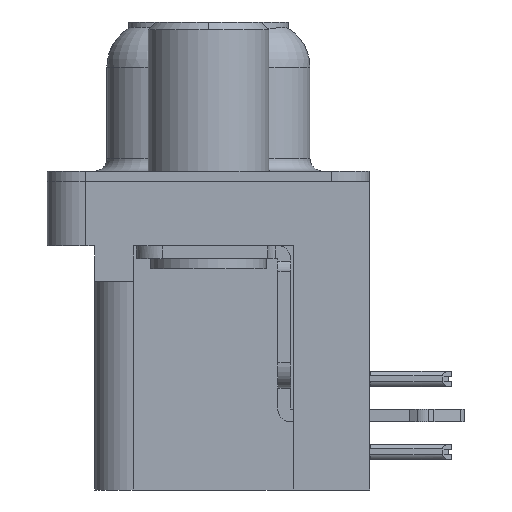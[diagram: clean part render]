
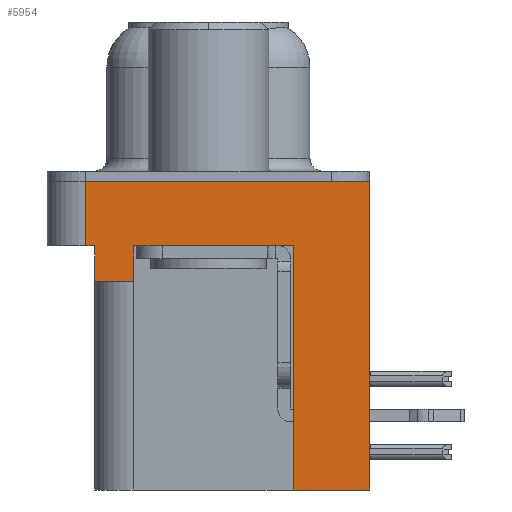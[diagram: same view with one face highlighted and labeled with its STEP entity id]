
A CAD part, left-side view. The second image highlights one B-rep face of the part: STEP entity #5954.
In plain terms, the highlighted planar face has unit normal (-1, 0, 0).
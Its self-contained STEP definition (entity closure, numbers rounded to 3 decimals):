
#320 = VECTOR ( 'NONE', #23377, 1000. ) ;
#1437 = VECTOR ( 'NONE', #6944, 1000. ) ;
#1944 = VECTOR ( 'NONE', #24552, 1000. ) ;
#2873 = AXIS2_PLACEMENT_3D ( 'NONE', #18936, #24991, #16897 ) ;
#3666 = VECTOR ( 'NONE', #25841, 1000. ) ;
#4092 = CARTESIAN_POINT ( 'NONE',  ( -2.935, -3.295, -12. ) ) ;
#4258 = VECTOR ( 'NONE', #9089, 1000. ) ;
#4611 = VECTOR ( 'NONE', #23401, 1000. ) ;
#4792 = EDGE_CURVE ( 'NONE', #22849, #14926, #17560, .T. ) ;
#5066 = VECTOR ( 'NONE', #19880, 1000. ) ;
#5247 = ORIENTED_EDGE ( 'NONE', *, *, #17541, .F. ) ;
#5258 = CARTESIAN_POINT ( 'NONE',  ( -2.935, 4.775, 0. ) ) ;
#5954 = ADVANCED_FACE ( 'NONE', ( #20139 ), #21109, .T. ) ;
#6425 = ORIENTED_EDGE ( 'NONE', *, *, #15629, .F. ) ;
#6846 = VERTEX_POINT ( 'NONE', #7409 ) ;
#6944 = DIRECTION ( 'NONE',  ( 0., 0., 1. ) ) ;
#7409 = CARTESIAN_POINT ( 'NONE',  ( -2.935, 4.425, -2.5 ) ) ;
#8389 = DIRECTION ( 'NONE',  ( 0., -1., 0. ) ) ;
#8557 = CARTESIAN_POINT ( 'NONE',  ( -2.935, -6.275, -12. ) ) ;
#9089 = DIRECTION ( 'NONE',  ( 0., 0., 1. ) ) ;
#9240 = ORIENTED_EDGE ( 'NONE', *, *, #19160, .T. ) ;
#9241 = CARTESIAN_POINT ( 'NONE',  ( -2.935, 4.425, -3.9 ) ) ;
#9741 = CARTESIAN_POINT ( 'NONE',  ( -2.935, -6.275, -2.5 ) ) ;
#9823 = DIRECTION ( 'NONE',  ( 0., 0., 1. ) ) ;
#10396 = ORIENTED_EDGE ( 'NONE', *, *, #18893, .T. ) ;
#10467 = CARTESIAN_POINT ( 'NONE',  ( -2.935, -6.275, 0. ) ) ;
#10673 = LINE ( 'NONE', #23793, #5066 ) ;
#10853 = CARTESIAN_POINT ( 'NONE',  ( -2.935, 2.895, -3.9 ) ) ;
#10885 = LINE ( 'NONE', #19027, #4611 ) ;
#11227 = ORIENTED_EDGE ( 'NONE', *, *, #20827, .F. ) ;
#11472 = LINE ( 'NONE', #19969, #1944 ) ;
#12484 = LINE ( 'NONE', #4092, #21060 ) ;
#12675 = CARTESIAN_POINT ( 'NONE',  ( -2.935, -6.275, 0. ) ) ;
#12857 = LINE ( 'NONE', #15121, #320 ) ;
#13091 = ORIENTED_EDGE ( 'NONE', *, *, #19710, .F. ) ;
#13749 = VECTOR ( 'NONE', #8389, 1000. ) ;
#14563 = DIRECTION ( 'NONE',  ( 0., 1., 0. ) ) ;
#14926 = VERTEX_POINT ( 'NONE', #24550 ) ;
#15121 = CARTESIAN_POINT ( 'NONE',  ( -2.935, -3.295, -12. ) ) ;
#15629 = EDGE_CURVE ( 'NONE', #22641, #6846, #24526, .T. ) ;
#16434 = LINE ( 'NONE', #12675, #13749 ) ;
#16897 = DIRECTION ( 'NONE',  ( 0., 0., 1. ) ) ;
#16963 = ORIENTED_EDGE ( 'NONE', *, *, #4792, .T. ) ;
#17541 = EDGE_CURVE ( 'NONE', #22849, #22641, #10885, .T. ) ;
#17560 = LINE ( 'NONE', #10853, #3666 ) ;
#17630 = VERTEX_POINT ( 'NONE', #10467 ) ;
#17770 = ORIENTED_EDGE ( 'NONE', *, *, #19288, .T. ) ;
#18009 = LINE ( 'NONE', #9741, #19653 ) ;
#18197 = EDGE_CURVE ( 'NONE', #25537, #19764, #12857, .T. ) ;
#18319 = VERTEX_POINT ( 'NONE', #5258 ) ;
#18652 = EDGE_CURVE ( 'NONE', #26982, #18319, #25738, .T. ) ;
#18893 = EDGE_CURVE ( 'NONE', #21520, #17630, #18009, .T. ) ;
#18936 = CARTESIAN_POINT ( 'NONE',  ( -2.935, -6.275, -2.5 ) ) ;
#19027 = CARTESIAN_POINT ( 'NONE',  ( -2.935, 4.425, -3.9 ) ) ;
#19160 = EDGE_CURVE ( 'NONE', #14926, #19764, #10673, .T. ) ;
#19288 = EDGE_CURVE ( 'NONE', #26982, #6846, #11472, .T. ) ;
#19653 = VECTOR ( 'NONE', #9823, 1000. ) ;
#19710 = EDGE_CURVE ( 'NONE', #21520, #25537, #12484, .T. ) ;
#19764 = VERTEX_POINT ( 'NONE', #22930 ) ;
#19880 = DIRECTION ( 'NONE',  ( 0., -1., 0. ) ) ;
#19969 = CARTESIAN_POINT ( 'NONE',  ( -2.935, -6.275, -2.5 ) ) ;
#20139 = FACE_OUTER_BOUND ( 'NONE', #22570, .T. ) ;
#20827 = EDGE_CURVE ( 'NONE', #18319, #17630, #16434, .T. ) ;
#21060 = VECTOR ( 'NONE', #14563, 1000. ) ;
#21109 = PLANE ( 'NONE',  #2873 ) ;
#21520 = VERTEX_POINT ( 'NONE', #8557 ) ;
#21771 = CARTESIAN_POINT ( 'NONE',  ( -2.935, 4.775, -2.5 ) ) ;
#22011 = ORIENTED_EDGE ( 'NONE', *, *, #18197, .F. ) ;
#22570 = EDGE_LOOP ( 'NONE', ( #11227, #24119, #17770, #6425, #5247, #16963, #9240, #22011, #13091, #10396 ) ) ;
#22641 = VERTEX_POINT ( 'NONE', #23588 ) ;
#22849 = VERTEX_POINT ( 'NONE', #23180 ) ;
#22930 = CARTESIAN_POINT ( 'NONE',  ( -2.935, -3.295, -2.5 ) ) ;
#23180 = CARTESIAN_POINT ( 'NONE',  ( -2.935, 2.895, -3.9 ) ) ;
#23377 = DIRECTION ( 'NONE',  ( 0., 0., 1. ) ) ;
#23401 = DIRECTION ( 'NONE',  ( 0., 1., 0. ) ) ;
#23588 = CARTESIAN_POINT ( 'NONE',  ( -2.935, 4.425, -3.9 ) ) ;
#23793 = CARTESIAN_POINT ( 'NONE',  ( -2.935, -6.275, -2.5 ) ) ;
#23990 = CARTESIAN_POINT ( 'NONE',  ( -2.935, 4.775, -2.5 ) ) ;
#24119 = ORIENTED_EDGE ( 'NONE', *, *, #18652, .F. ) ;
#24526 = LINE ( 'NONE', #9241, #1437 ) ;
#24550 = CARTESIAN_POINT ( 'NONE',  ( -2.935, 2.895, -2.5 ) ) ;
#24552 = DIRECTION ( 'NONE',  ( 0., -1., 0. ) ) ;
#24991 = DIRECTION ( 'NONE',  ( -1., 0., 0. ) ) ;
#25445 = CARTESIAN_POINT ( 'NONE',  ( -2.935, -3.295, -12. ) ) ;
#25537 = VERTEX_POINT ( 'NONE', #25445 ) ;
#25738 = LINE ( 'NONE', #21771, #4258 ) ;
#25841 = DIRECTION ( 'NONE',  ( 0., 0., 1. ) ) ;
#26982 = VERTEX_POINT ( 'NONE', #23990 ) ;
